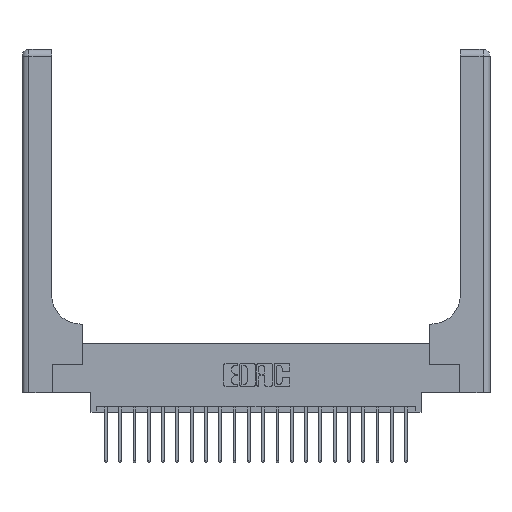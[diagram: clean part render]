
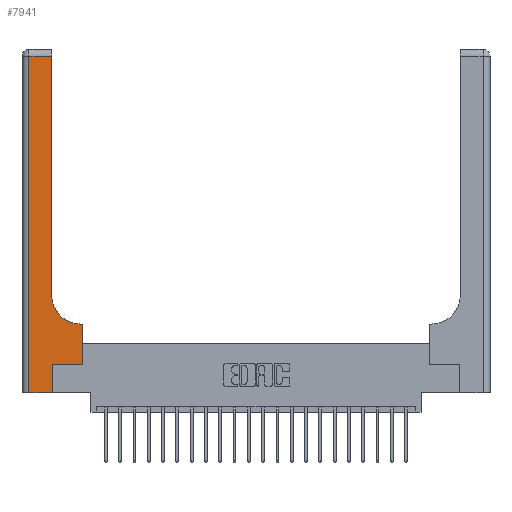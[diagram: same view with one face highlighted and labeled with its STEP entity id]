
A CAD part, top view. The second image highlights one B-rep face of the part: STEP entity #7941.
In plain terms, the highlighted planar face has unit normal (0, 0, 1).
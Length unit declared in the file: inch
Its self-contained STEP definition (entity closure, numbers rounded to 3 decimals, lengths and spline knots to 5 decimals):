
#1441 = CARTESIAN_POINT ( 'NONE',  ( 0.51, 0.85, 0.37 ) ) ;
#1476 = VERTEX_POINT ( 'NONE', #13399 ) ;
#1675 = VERTEX_POINT ( 'NONE', #12273 ) ;
#1801 = CARTESIAN_POINT ( 'NONE',  ( 0.06, 3., 0.37 ) ) ;
#1844 = CARTESIAN_POINT ( 'NONE',  ( 0.265, 0.25, 0.37 ) ) ;
#2101 = VECTOR ( 'NONE', #9248, 39.37008 ) ;
#2967 = CARTESIAN_POINT ( 'NONE',  ( 0.528, 0.25, 0.37 ) ) ;
#3178 = DIRECTION ( 'NONE',  ( 1., 0., 0. ) ) ;
#3982 = CARTESIAN_POINT ( 'NONE',  ( 0.51, 0.6, 0.37 ) ) ;
#4188 = LINE ( 'NONE', #19439, #13408 ) ;
#4252 = VERTEX_POINT ( 'NONE', #7154 ) ;
#4745 = CARTESIAN_POINT ( 'NONE',  ( 0.26, 2.94, 0.37 ) ) ;
#5327 = ORIENTED_EDGE ( 'NONE', *, *, #7015, .T. ) ;
#5693 = DIRECTION ( 'NONE',  ( -1., 0., 0. ) ) ;
#5988 = LINE ( 'NONE', #21098, #9487 ) ;
#6209 = LINE ( 'NONE', #10296, #10812 ) ;
#6421 = ORIENTED_EDGE ( 'NONE', *, *, #10961, .T. ) ;
#6470 = DIRECTION ( 'NONE',  ( 0., 0., -1. ) ) ;
#6561 = VECTOR ( 'NONE', #16044, 39.37008 ) ;
#7015 = EDGE_CURVE ( 'NONE', #10200, #20877, #9608, .T. ) ;
#7154 = CARTESIAN_POINT ( 'NONE',  ( 0.528, 0.25, 0.37 ) ) ;
#7941 = ADVANCED_FACE ( 'NONE', ( #15076 ), #15018, .F. ) ;
#7957 = AXIS2_PLACEMENT_3D ( 'NONE', #16803, #6470, #18569 ) ;
#8934 = EDGE_CURVE ( 'NONE', #19826, #18069, #4188, .T. ) ;
#9068 = VECTOR ( 'NONE', #15131, 39.37008 ) ;
#9070 = VECTOR ( 'NONE', #5693, 39.37008 ) ;
#9248 = DIRECTION ( 'NONE',  ( 0., 1., 0. ) ) ;
#9487 = VECTOR ( 'NONE', #10802, 39.37008 ) ;
#9608 = LINE ( 'NONE', #16018, #9070 ) ;
#9656 = ORIENTED_EDGE ( 'NONE', *, *, #20161, .T. ) ;
#10200 = VERTEX_POINT ( 'NONE', #4745 ) ;
#10296 = CARTESIAN_POINT ( 'NONE',  ( 0.26, 0.6, 0.37 ) ) ;
#10802 = DIRECTION ( 'NONE',  ( 0., 1., 0. ) ) ;
#10812 = VECTOR ( 'NONE', #18929, 39.37008 ) ;
#10961 = EDGE_CURVE ( 'NONE', #14976, #4252, #20324, .T. ) ;
#10986 = CARTESIAN_POINT ( 'NONE',  ( 0.26, 3., 0.37 ) ) ;
#11549 = LINE ( 'NONE', #1801, #16117 ) ;
#12237 = DIRECTION ( 'NONE',  ( 0., -1., 0. ) ) ;
#12273 = CARTESIAN_POINT ( 'NONE',  ( 0.528, 0.6, 0.37 ) ) ;
#13121 = LINE ( 'NONE', #2967, #9068 ) ;
#13399 = CARTESIAN_POINT ( 'NONE',  ( 0.26, 0.85, 0.37 ) ) ;
#13408 = VECTOR ( 'NONE', #17680, 39.37008 ) ;
#13468 = ORIENTED_EDGE ( 'NONE', *, *, #14089, .T. ) ;
#13487 = EDGE_CURVE ( 'NONE', #1675, #15106, #6209, .T. ) ;
#13580 = DIRECTION ( 'NONE',  ( 0., 0., -1. ) ) ;
#14089 = EDGE_CURVE ( 'NONE', #15106, #1476, #17800, .T. ) ;
#14313 = CARTESIAN_POINT ( 'NONE',  ( 0.265, 0.25, 0.37 ) ) ;
#14462 = CARTESIAN_POINT ( 'NONE',  ( 0.265, 0., 0.37 ) ) ;
#14796 = ORIENTED_EDGE ( 'NONE', *, *, #8934, .T. ) ;
#14947 = EDGE_LOOP ( 'NONE', ( #18552, #5327, #9656, #14796, #17493, #6421, #19424, #22052, #13468 ) ) ;
#14976 = VERTEX_POINT ( 'NONE', #1844 ) ;
#15018 = PLANE ( 'NONE',  #7957 ) ;
#15076 = FACE_OUTER_BOUND ( 'NONE', #14947, .T. ) ;
#15106 = VERTEX_POINT ( 'NONE', #3982 ) ;
#15131 = DIRECTION ( 'NONE',  ( 0., 1., 0. ) ) ;
#15934 = LINE ( 'NONE', #10986, #2101 ) ;
#16018 = CARTESIAN_POINT ( 'NONE',  ( 0., 2.94, 0.37 ) ) ;
#16044 = DIRECTION ( 'NONE',  ( 1., 0., 0. ) ) ;
#16117 = VECTOR ( 'NONE', #12237, 39.37008 ) ;
#16214 = CARTESIAN_POINT ( 'NONE',  ( 0.06, 0., 0.37 ) ) ;
#16803 = CARTESIAN_POINT ( 'NONE',  ( 0., 3., 0.37 ) ) ;
#17493 = ORIENTED_EDGE ( 'NONE', *, *, #21315, .T. ) ;
#17680 = DIRECTION ( 'NONE',  ( 1., 0., 0. ) ) ;
#17800 = CIRCLE ( 'NONE', #19211, 0.25 ) ;
#18038 = EDGE_CURVE ( 'NONE', #1476, #10200, #15934, .T. ) ;
#18069 = VERTEX_POINT ( 'NONE', #14462 ) ;
#18552 = ORIENTED_EDGE ( 'NONE', *, *, #18038, .T. ) ;
#18569 = DIRECTION ( 'NONE',  ( -1., 0., 0. ) ) ;
#18929 = DIRECTION ( 'NONE',  ( -1., 0., 0. ) ) ;
#19211 = AXIS2_PLACEMENT_3D ( 'NONE', #1441, #13580, #3178 ) ;
#19424 = ORIENTED_EDGE ( 'NONE', *, *, #21037, .T. ) ;
#19439 = CARTESIAN_POINT ( 'NONE',  ( 0., 0., 0.37 ) ) ;
#19826 = VERTEX_POINT ( 'NONE', #16214 ) ;
#20161 = EDGE_CURVE ( 'NONE', #20877, #19826, #11549, .T. ) ;
#20324 = LINE ( 'NONE', #14313, #6561 ) ;
#20877 = VERTEX_POINT ( 'NONE', #21336 ) ;
#21037 = EDGE_CURVE ( 'NONE', #4252, #1675, #13121, .T. ) ;
#21098 = CARTESIAN_POINT ( 'NONE',  ( 0.265, 0., 0.37 ) ) ;
#21315 = EDGE_CURVE ( 'NONE', #18069, #14976, #5988, .T. ) ;
#21336 = CARTESIAN_POINT ( 'NONE',  ( 0.06, 2.94, 0.37 ) ) ;
#22052 = ORIENTED_EDGE ( 'NONE', *, *, #13487, .T. ) ;
